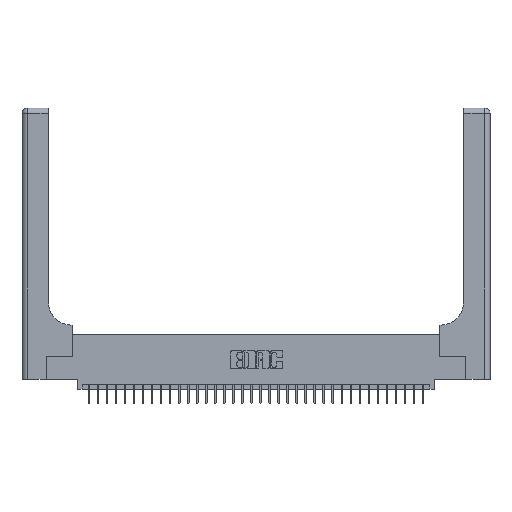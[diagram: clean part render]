
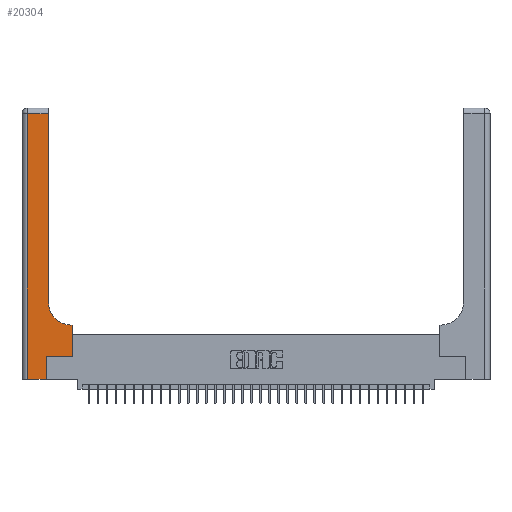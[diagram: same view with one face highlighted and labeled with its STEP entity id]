
A CAD part, top view. The second image highlights one B-rep face of the part: STEP entity #20304.
In plain terms, the highlighted planar face has unit normal (0, 0, 1).
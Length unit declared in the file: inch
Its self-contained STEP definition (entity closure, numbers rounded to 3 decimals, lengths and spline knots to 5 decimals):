
#868 = LINE ( 'NONE', #25464, #16552 ) ;
#965 = VERTEX_POINT ( 'NONE', #24926 ) ;
#1386 = CARTESIAN_POINT ( 'NONE',  ( 0.5585, 0.25, 0.37 ) ) ;
#1433 = DIRECTION ( 'NONE',  ( 0., 1., 0. ) ) ;
#1731 = EDGE_CURVE ( 'NONE', #9760, #3272, #30414, .T. ) ;
#2041 = DIRECTION ( 'NONE',  ( 0., 0., -1. ) ) ;
#2300 = LINE ( 'NONE', #1386, #30783 ) ;
#2340 = VERTEX_POINT ( 'NONE', #28312 ) ;
#2418 = ORIENTED_EDGE ( 'NONE', *, *, #20248, .T. ) ;
#2588 = CARTESIAN_POINT ( 'NONE',  ( 0.269, 0.25, 0.37 ) ) ;
#3029 = VECTOR ( 'NONE', #23299, 39.37008 ) ;
#3272 = VERTEX_POINT ( 'NONE', #16149 ) ;
#3593 = ORIENTED_EDGE ( 'NONE', *, *, #1731, .T. ) ;
#4837 = CARTESIAN_POINT ( 'NONE',  ( 0.2915, 2.94, 0.37 ) ) ;
#6024 = AXIS2_PLACEMENT_3D ( 'NONE', #23050, #6559, #25785 ) ;
#6559 = DIRECTION ( 'NONE',  ( 0., 0., -1. ) ) ;
#8102 = CARTESIAN_POINT ( 'NONE',  ( 0., 2.94, 0.37 ) ) ;
#8560 = VECTOR ( 'NONE', #17820, 39.37008 ) ;
#8991 = AXIS2_PLACEMENT_3D ( 'NONE', #12793, #2041, #21427 ) ;
#9514 = CARTESIAN_POINT ( 'NONE',  ( 0.269, 0.25, 0.37 ) ) ;
#9760 = VERTEX_POINT ( 'NONE', #23293 ) ;
#9918 = CARTESIAN_POINT ( 'NONE',  ( 0.2915, 0.85, 0.37 ) ) ;
#10366 = FACE_OUTER_BOUND ( 'NONE', #19929, .T. ) ;
#10513 = LINE ( 'NONE', #9514, #3029 ) ;
#10664 = EDGE_CURVE ( 'NONE', #11250, #24948, #27910, .T. ) ;
#11250 = VERTEX_POINT ( 'NONE', #4837 ) ;
#11452 = CARTESIAN_POINT ( 'NONE',  ( 0., 0., 0.37 ) ) ;
#12036 = EDGE_CURVE ( 'NONE', #2340, #26109, #29519, .T. ) ;
#12793 = CARTESIAN_POINT ( 'NONE',  ( 0., 3., 0.37 ) ) ;
#13404 = DIRECTION ( 'NONE',  ( -1., 0., 0. ) ) ;
#13429 = VERTEX_POINT ( 'NONE', #28412 ) ;
#13443 = EDGE_CURVE ( 'NONE', #3272, #21246, #27995, .T. ) ;
#13905 = VECTOR ( 'NONE', #33453, 39.37008 ) ;
#14453 = DIRECTION ( 'NONE',  ( 0., -1., 0. ) ) ;
#15962 = ORIENTED_EDGE ( 'NONE', *, *, #10664, .T. ) ;
#16149 = CARTESIAN_POINT ( 'NONE',  ( 0.5415, 0.6, 0.37 ) ) ;
#16278 = EDGE_CURVE ( 'NONE', #13429, #9760, #2300, .T. ) ;
#16552 = VECTOR ( 'NONE', #14453, 39.37008 ) ;
#17820 = DIRECTION ( 'NONE',  ( -1., 0., 0. ) ) ;
#19929 = EDGE_LOOP ( 'NONE', ( #2418, #15962, #23599, #26255, #23271, #32411, #32880, #3593, #33605 ) ) ;
#20248 = EDGE_CURVE ( 'NONE', #21246, #11250, #33094, .T. ) ;
#20304 = ADVANCED_FACE ( 'NONE', ( #10366 ), #35105, .F. ) ;
#21246 = VERTEX_POINT ( 'NONE', #9918 ) ;
#21427 = DIRECTION ( 'NONE',  ( -1., 0., 0. ) ) ;
#21631 = EDGE_CURVE ( 'NONE', #965, #2340, #28261, .T. ) ;
#22426 = CARTESIAN_POINT ( 'NONE',  ( 0.269, 0., 0.37 ) ) ;
#23050 = CARTESIAN_POINT ( 'NONE',  ( 0.5415, 0.85, 0.37 ) ) ;
#23271 = ORIENTED_EDGE ( 'NONE', *, *, #12036, .T. ) ;
#23293 = CARTESIAN_POINT ( 'NONE',  ( 0.5585, 0.6, 0.37 ) ) ;
#23299 = DIRECTION ( 'NONE',  ( 1., 0., 0. ) ) ;
#23599 = ORIENTED_EDGE ( 'NONE', *, *, #35233, .T. ) ;
#24926 = CARTESIAN_POINT ( 'NONE',  ( 0.06, 0., 0.37 ) ) ;
#24948 = VERTEX_POINT ( 'NONE', #30407 ) ;
#25464 = CARTESIAN_POINT ( 'NONE',  ( 0.06, 3., 0.37 ) ) ;
#25689 = VECTOR ( 'NONE', #27839, 39.37008 ) ;
#25719 = EDGE_CURVE ( 'NONE', #26109, #13429, #10513, .T. ) ;
#25784 = VECTOR ( 'NONE', #1433, 39.37008 ) ;
#25785 = DIRECTION ( 'NONE',  ( 1., 0., 0. ) ) ;
#25959 = CARTESIAN_POINT ( 'NONE',  ( 0.2915, 0.6, 0.37 ) ) ;
#26109 = VERTEX_POINT ( 'NONE', #2588 ) ;
#26255 = ORIENTED_EDGE ( 'NONE', *, *, #21631, .T. ) ;
#27839 = DIRECTION ( 'NONE',  ( 1., 0., 0. ) ) ;
#27910 = LINE ( 'NONE', #8102, #35239 ) ;
#27995 = CIRCLE ( 'NONE', #6024, 0.25 ) ;
#28261 = LINE ( 'NONE', #11452, #25689 ) ;
#28312 = CARTESIAN_POINT ( 'NONE',  ( 0.269, 0., 0.37 ) ) ;
#28412 = CARTESIAN_POINT ( 'NONE',  ( 0.5585, 0.25, 0.37 ) ) ;
#28964 = CARTESIAN_POINT ( 'NONE',  ( 0.2915, 3., 0.37 ) ) ;
#29519 = LINE ( 'NONE', #22426, #13905 ) ;
#30407 = CARTESIAN_POINT ( 'NONE',  ( 0.06, 2.94, 0.37 ) ) ;
#30414 = LINE ( 'NONE', #25959, #8560 ) ;
#30783 = VECTOR ( 'NONE', #34578, 39.37008 ) ;
#32411 = ORIENTED_EDGE ( 'NONE', *, *, #25719, .T. ) ;
#32880 = ORIENTED_EDGE ( 'NONE', *, *, #16278, .T. ) ;
#33094 = LINE ( 'NONE', #28964, #25784 ) ;
#33453 = DIRECTION ( 'NONE',  ( 0., 1., 0. ) ) ;
#33605 = ORIENTED_EDGE ( 'NONE', *, *, #13443, .T. ) ;
#34578 = DIRECTION ( 'NONE',  ( 0., 1., 0. ) ) ;
#35105 = PLANE ( 'NONE',  #8991 ) ;
#35233 = EDGE_CURVE ( 'NONE', #24948, #965, #868, .T. ) ;
#35239 = VECTOR ( 'NONE', #13404, 39.37008 ) ;
